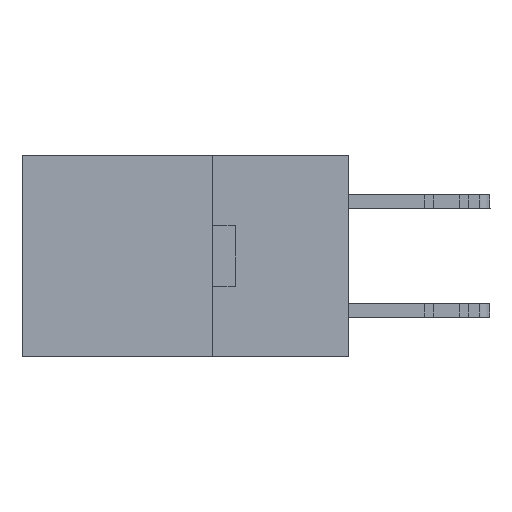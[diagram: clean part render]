
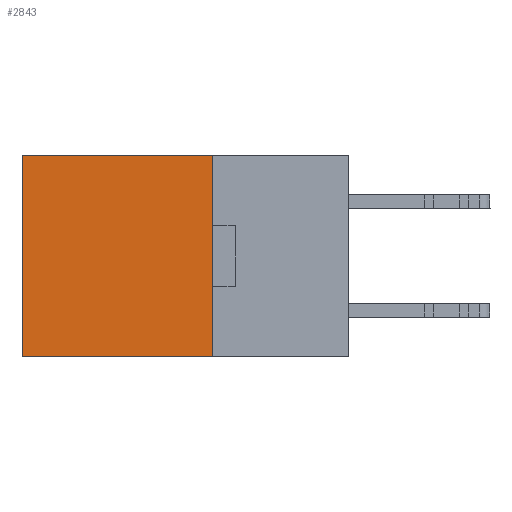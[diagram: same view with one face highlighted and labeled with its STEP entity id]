
A CAD part, left-side view. The second image highlights one B-rep face of the part: STEP entity #2843.
In plain terms, the highlighted planar face has unit normal (-1, 0, 0).
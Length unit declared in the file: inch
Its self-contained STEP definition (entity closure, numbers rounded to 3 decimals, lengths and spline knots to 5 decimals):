
#2387 = CARTESIAN_POINT ( 'NONE',  ( 0.2615, 0.25, -0.37 ) ) ;
#2645 = EDGE_CURVE ( 'NONE', #19748, #16953, #24077, .T. ) ;
#2843 = ADVANCED_FACE ( 'NONE', ( #7982 ), #25851, .F. ) ;
#3334 = CARTESIAN_POINT ( 'NONE',  ( 0.2615, 0.25, -0.37 ) ) ;
#3913 = CARTESIAN_POINT ( 'NONE',  ( 0.2615, 0.25, 0. ) ) ;
#4014 = VECTOR ( 'NONE', #24650, 39.37008 ) ;
#4171 = EDGE_CURVE ( 'NONE', #16953, #11952, #9892, .T. ) ;
#6886 = DIRECTION ( 'NONE',  ( 0., 0., -1. ) ) ;
#6972 = VECTOR ( 'NONE', #10237, 39.37008 ) ;
#7133 = CARTESIAN_POINT ( 'NONE',  ( 0.2615, 0.25, 0. ) ) ;
#7982 = FACE_OUTER_BOUND ( 'NONE', #26046, .T. ) ;
#8302 = EDGE_CURVE ( 'NONE', #19748, #24557, #15586, .T. ) ;
#8844 = DIRECTION ( 'NONE',  ( 0., 0., -1. ) ) ;
#9691 = EDGE_CURVE ( 'NONE', #24557, #11952, #19758, .T. ) ;
#9892 = LINE ( 'NONE', #23471, #20635 ) ;
#10237 = DIRECTION ( 'NONE',  ( 0., 1., 0. ) ) ;
#11952 = VERTEX_POINT ( 'NONE', #27161 ) ;
#13592 = CARTESIAN_POINT ( 'NONE',  ( 0.2615, 0.6, 0. ) ) ;
#14388 = CARTESIAN_POINT ( 'NONE',  ( 0.2615, 0.25, -0.37 ) ) ;
#15586 = LINE ( 'NONE', #21851, #20602 ) ;
#16497 = ORIENTED_EDGE ( 'NONE', *, *, #2645, .T. ) ;
#16953 = VERTEX_POINT ( 'NONE', #13592 ) ;
#17080 = AXIS2_PLACEMENT_3D ( 'NONE', #2387, #21648, #8844 ) ;
#19351 = ORIENTED_EDGE ( 'NONE', *, *, #4171, .T. ) ;
#19568 = ORIENTED_EDGE ( 'NONE', *, *, #9691, .F. ) ;
#19748 = VERTEX_POINT ( 'NONE', #7133 ) ;
#19758 = LINE ( 'NONE', #3334, #4014 ) ;
#20602 = VECTOR ( 'NONE', #6886, 39.37008 ) ;
#20635 = VECTOR ( 'NONE', #21400, 39.37008 ) ;
#21400 = DIRECTION ( 'NONE',  ( 0., 0., -1. ) ) ;
#21648 = DIRECTION ( 'NONE',  ( 1., 0., 0. ) ) ;
#21851 = CARTESIAN_POINT ( 'NONE',  ( 0.2615, 0.25, -0.37 ) ) ;
#23471 = CARTESIAN_POINT ( 'NONE',  ( 0.2615, 0.6, -0.37 ) ) ;
#24077 = LINE ( 'NONE', #3913, #6972 ) ;
#24350 = ORIENTED_EDGE ( 'NONE', *, *, #8302, .F. ) ;
#24557 = VERTEX_POINT ( 'NONE', #14388 ) ;
#24650 = DIRECTION ( 'NONE',  ( 0., 1., 0. ) ) ;
#25851 = PLANE ( 'NONE',  #17080 ) ;
#26046 = EDGE_LOOP ( 'NONE', ( #19351, #19568, #24350, #16497 ) ) ;
#27161 = CARTESIAN_POINT ( 'NONE',  ( 0.2615, 0.6, -0.37 ) ) ;
